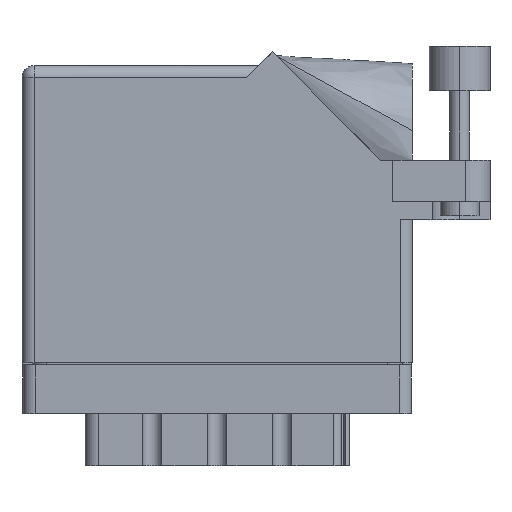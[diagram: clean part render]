
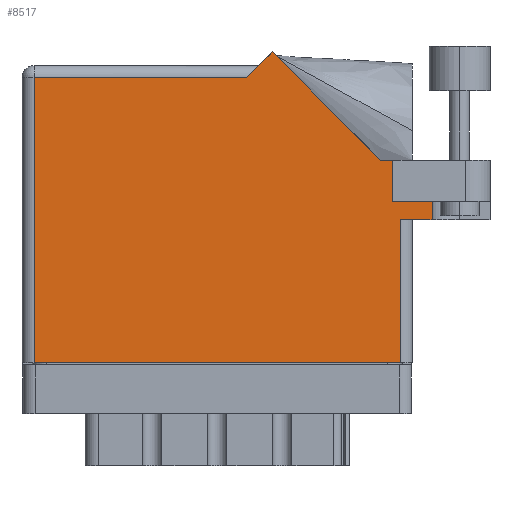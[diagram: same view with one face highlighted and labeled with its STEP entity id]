
A CAD part, front view. The second image highlights one B-rep face of the part: STEP entity #8517.
In plain terms, the highlighted face is planar.
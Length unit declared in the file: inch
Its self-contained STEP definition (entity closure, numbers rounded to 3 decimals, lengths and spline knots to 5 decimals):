
#413 = VECTOR ( 'NONE', #28916, 39.37008 ) ;
#520 = CARTESIAN_POINT ( 'NONE',  ( 1.84442, 1.044, 0. ) ) ;
#762 = CARTESIAN_POINT ( 'NONE',  ( 2.01, 0.737, 0. ) ) ;
#767 = VERTEX_POINT ( 'NONE', #3359 ) ;
#1453 = CARTESIAN_POINT ( 'NONE',  ( 0.062, 0., 0. ) ) ;
#1596 = ORIENTED_EDGE ( 'NONE', *, *, #3955, .T. ) ;
#1786 = CARTESIAN_POINT ( 'NONE',  ( 2.1115, 0.737, 0. ) ) ;
#2419 = DIRECTION ( 'NONE',  ( -1., 0., 0. ) ) ;
#2918 = CARTESIAN_POINT ( 'NONE',  ( 0., 1.468, 0. ) ) ;
#3359 = CARTESIAN_POINT ( 'NONE',  ( 2.1115, 0.831, 0. ) ) ;
#3894 = DIRECTION ( 'NONE',  ( 0., 1., 0. ) ) ;
#3955 = EDGE_CURVE ( 'NONE', #21775, #14311, #11186, .T. ) ;
#4080 = ORIENTED_EDGE ( 'NONE', *, *, #35431, .T. ) ;
#4125 = VERTEX_POINT ( 'NONE', #29592 ) ;
#4736 = LINE ( 'NONE', #30144, #29389 ) ;
#6618 = VERTEX_POINT ( 'NONE', #18820 ) ;
#6798 = VECTOR ( 'NONE', #2419, 39.37008 ) ;
#6803 = LINE ( 'NONE', #10360, #23716 ) ;
#7194 = FACE_OUTER_BOUND ( 'NONE', #8454, .T. ) ;
#7299 = LINE ( 'NONE', #762, #11330 ) ;
#7688 = LINE ( 'NONE', #1453, #17706 ) ;
#8454 = EDGE_LOOP ( 'NONE', ( #10390, #9394, #36313, #33710, #32731, #18177, #4080, #22750, #36542, #1596, #30761 ) ) ;
#8517 = ADVANCED_FACE ( 'NONE', ( #7194 ), #38787, .F. ) ;
#8656 = CARTESIAN_POINT ( 'NONE',  ( 1.217, 1.53, 0. ) ) ;
#8677 = DIRECTION ( 'NONE',  ( 0., 1., 0. ) ) ;
#8874 = LINE ( 'NONE', #31975, #9856 ) ;
#8983 = LINE ( 'NONE', #22858, #413 ) ;
#9077 = DIRECTION ( 'NONE',  ( -0.707, -0.707, 0. ) ) ;
#9205 = VERTEX_POINT ( 'NONE', #19792 ) ;
#9394 = ORIENTED_EDGE ( 'NONE', *, *, #18530, .T. ) ;
#9856 = VECTOR ( 'NONE', #38600, 39.37008 ) ;
#9987 = VERTEX_POINT ( 'NONE', #520 ) ;
#10125 = CARTESIAN_POINT ( 'NONE',  ( 1.28771, 1.60071, 0. ) ) ;
#10343 = EDGE_CURVE ( 'NONE', #22523, #21775, #27727, .T. ) ;
#10360 = CARTESIAN_POINT ( 'NONE',  ( 1.948, 0.737, 0. ) ) ;
#10379 = CARTESIAN_POINT ( 'NONE',  ( 0.062, 1.468, 0. ) ) ;
#10390 = ORIENTED_EDGE ( 'NONE', *, *, #13584, .T. ) ;
#11186 = LINE ( 'NONE', #2918, #14687 ) ;
#11330 = VECTOR ( 'NONE', #29838, 39.37008 ) ;
#13584 = EDGE_CURVE ( 'NONE', #4125, #24318, #4736, .T. ) ;
#13943 = VECTOR ( 'NONE', #8677, 39.37008 ) ;
#14311 = VERTEX_POINT ( 'NONE', #10379 ) ;
#14576 = VERTEX_POINT ( 'NONE', #1786 ) ;
#14687 = VECTOR ( 'NONE', #38484, 39.37008 ) ;
#17217 = DIRECTION ( 'NONE',  ( 0., 0., -1. ) ) ;
#17706 = VECTOR ( 'NONE', #37016, 39.37008 ) ;
#18177 = ORIENTED_EDGE ( 'NONE', *, *, #30217, .T. ) ;
#18424 = CARTESIAN_POINT ( 'NONE',  ( 2.41, 1.044, 0. ) ) ;
#18497 = CARTESIAN_POINT ( 'NONE',  ( 1.155, 1.468, 0. ) ) ;
#18530 = EDGE_CURVE ( 'NONE', #24318, #6618, #6803, .T. ) ;
#18563 = VECTOR ( 'NONE', #37446, 39.37008 ) ;
#18820 = CARTESIAN_POINT ( 'NONE',  ( 1.948, 0.737, 0. ) ) ;
#19792 = CARTESIAN_POINT ( 'NONE',  ( 1.91, 0.831, 0. ) ) ;
#20313 = DIRECTION ( 'NONE',  ( -1., 0., 0. ) ) ;
#20349 = EDGE_CURVE ( 'NONE', #14311, #4125, #7688, .T. ) ;
#21775 = VERTEX_POINT ( 'NONE', #18497 ) ;
#22356 = EDGE_CURVE ( 'NONE', #9205, #767, #31142, .T. ) ;
#22510 = LINE ( 'NONE', #37511, #13943 ) ;
#22523 = VERTEX_POINT ( 'NONE', #10125 ) ;
#22750 = ORIENTED_EDGE ( 'NONE', *, *, #33812, .T. ) ;
#22858 = CARTESIAN_POINT ( 'NONE',  ( 2.1115, 1.16177, 0. ) ) ;
#22876 = LINE ( 'NONE', #18424, #6798 ) ;
#23609 = CARTESIAN_POINT ( 'NONE',  ( 1.948, 0., 0. ) ) ;
#23716 = VECTOR ( 'NONE', #3894, 39.37008 ) ;
#24318 = VERTEX_POINT ( 'NONE', #23609 ) ;
#24485 = CARTESIAN_POINT ( 'NONE',  ( 1.91, 0.831, 0. ) ) ;
#25497 = EDGE_CURVE ( 'NONE', #6618, #14576, #7299, .T. ) ;
#26233 = VECTOR ( 'NONE', #9077, 39.37008 ) ;
#27727 = LINE ( 'NONE', #8656, #26233 ) ;
#27892 = VERTEX_POINT ( 'NONE', #38119 ) ;
#28916 = DIRECTION ( 'NONE',  ( 0., -1., 0. ) ) ;
#29389 = VECTOR ( 'NONE', #30275, 39.37008 ) ;
#29592 = CARTESIAN_POINT ( 'NONE',  ( 0.062, 0., 0. ) ) ;
#29838 = DIRECTION ( 'NONE',  ( 1., 0., 0. ) ) ;
#29886 = EDGE_CURVE ( 'NONE', #767, #14576, #8983, .T. ) ;
#30144 = CARTESIAN_POINT ( 'NONE',  ( 0., 0., 0. ) ) ;
#30217 = EDGE_CURVE ( 'NONE', #9205, #27892, #22510, .T. ) ;
#30275 = DIRECTION ( 'NONE',  ( 1., 0., 0. ) ) ;
#30761 = ORIENTED_EDGE ( 'NONE', *, *, #20349, .T. ) ;
#31142 = LINE ( 'NONE', #24485, #18563 ) ;
#31465 = AXIS2_PLACEMENT_3D ( 'NONE', #39773, #17217, #20313 ) ;
#31975 = CARTESIAN_POINT ( 'NONE',  ( 1.84442, 1.044, 0. ) ) ;
#32731 = ORIENTED_EDGE ( 'NONE', *, *, #22356, .F. ) ;
#33710 = ORIENTED_EDGE ( 'NONE', *, *, #29886, .F. ) ;
#33812 = EDGE_CURVE ( 'NONE', #9987, #22523, #8874, .T. ) ;
#35431 = EDGE_CURVE ( 'NONE', #27892, #9987, #22876, .T. ) ;
#36313 = ORIENTED_EDGE ( 'NONE', *, *, #25497, .T. ) ;
#36542 = ORIENTED_EDGE ( 'NONE', *, *, #10343, .T. ) ;
#37016 = DIRECTION ( 'NONE',  ( 0., -1., 0. ) ) ;
#37446 = DIRECTION ( 'NONE',  ( 1., 0., 0. ) ) ;
#37511 = CARTESIAN_POINT ( 'NONE',  ( 1.91, 0.831, 0. ) ) ;
#38119 = CARTESIAN_POINT ( 'NONE',  ( 1.91, 1.044, 0. ) ) ;
#38484 = DIRECTION ( 'NONE',  ( -1., 0., 0. ) ) ;
#38600 = DIRECTION ( 'NONE',  ( -0.707, 0.707, 0. ) ) ;
#38787 = PLANE ( 'NONE',  #31465 ) ;
#39773 = CARTESIAN_POINT ( 'NONE',  ( 0., 1.53, 0. ) ) ;
